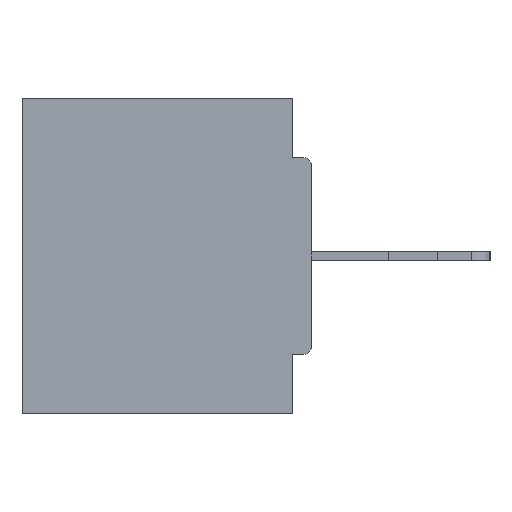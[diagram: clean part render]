
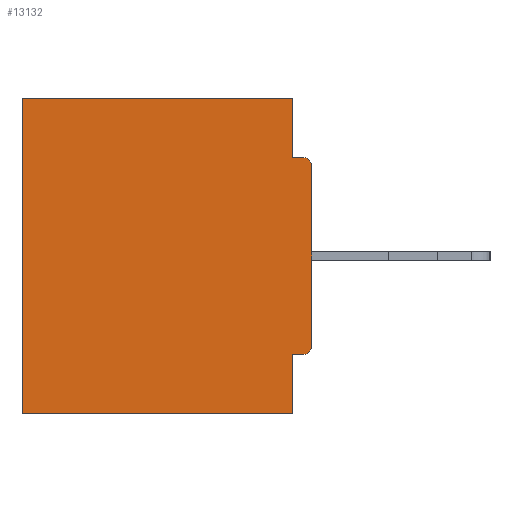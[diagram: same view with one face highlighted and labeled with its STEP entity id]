
A CAD part, left-side view. The second image highlights one B-rep face of the part: STEP entity #13132.
In plain terms, the highlighted planar face has unit normal (-1, 0, 0).
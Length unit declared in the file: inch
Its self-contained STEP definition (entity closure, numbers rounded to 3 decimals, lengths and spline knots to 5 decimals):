
#302 = DIRECTION ( 'NONE',  ( 0., 0., -1. ) ) ;
#1780 = VERTEX_POINT ( 'NONE', #10570 ) ;
#2366 = VERTEX_POINT ( 'NONE', #28621 ) ;
#2694 = LINE ( 'NONE', #25686, #20360 ) ;
#2713 = DIRECTION ( 'NONE',  ( 0., 0., -1. ) ) ;
#3086 = ORIENTED_EDGE ( 'NONE', *, *, #17525, .T. ) ;
#3240 = CARTESIAN_POINT ( 'NONE',  ( 0.298, 0.015, -0.1085 ) ) ;
#3251 = ORIENTED_EDGE ( 'NONE', *, *, #28039, .F. ) ;
#4058 = ORIENTED_EDGE ( 'NONE', *, *, #23724, .F. ) ;
#5071 = CARTESIAN_POINT ( 'NONE',  ( 0.298, 0.031, -0.5 ) ) ;
#5404 = EDGE_CURVE ( 'NONE', #2366, #26169, #7298, .T. ) ;
#5923 = AXIS2_PLACEMENT_3D ( 'NONE', #3240, #13696, #24022 ) ;
#6065 = CARTESIAN_POINT ( 'NONE',  ( 0.298, 0.46, 0. ) ) ;
#6182 = VECTOR ( 'NONE', #30196, 39.37008 ) ;
#6860 = LINE ( 'NONE', #17174, #6182 ) ;
#6928 = CARTESIAN_POINT ( 'NONE',  ( 0.298, 0., -0.3915 ) ) ;
#7298 = LINE ( 'NONE', #27934, #16005 ) ;
#7445 = VERTEX_POINT ( 'NONE', #14035 ) ;
#7808 = VERTEX_POINT ( 'NONE', #9092 ) ;
#9092 = CARTESIAN_POINT ( 'NONE',  ( 0.298, 0.015, -0.4065 ) ) ;
#9270 = CIRCLE ( 'NONE', #23283, 0.015 ) ;
#10570 = CARTESIAN_POINT ( 'NONE',  ( 0.298, 0.031, -0.0935 ) ) ;
#10773 = DIRECTION ( 'NONE',  ( 0., 1., 0. ) ) ;
#11004 = ORIENTED_EDGE ( 'NONE', *, *, #5404, .F. ) ;
#11355 = ORIENTED_EDGE ( 'NONE', *, *, #17517, .T. ) ;
#12876 = DIRECTION ( 'NONE',  ( 0., 0., -1. ) ) ;
#13080 = CARTESIAN_POINT ( 'NONE',  ( 0.298, 0., -0.0935 ) ) ;
#13132 = ADVANCED_FACE ( 'NONE', ( #18272 ), #18106, .F. ) ;
#13502 = VERTEX_POINT ( 'NONE', #6928 ) ;
#13691 = EDGE_CURVE ( 'NONE', #7445, #24953, #26862, .T. ) ;
#13696 = DIRECTION ( 'NONE',  ( -1., 0., 0. ) ) ;
#13926 = CARTESIAN_POINT ( 'NONE',  ( 0.298, 0., -0.1085 ) ) ;
#14035 = CARTESIAN_POINT ( 'NONE',  ( 0.298, 0.46, 0. ) ) ;
#15209 = VECTOR ( 'NONE', #10773, 39.37008 ) ;
#15404 = DIRECTION ( 'NONE',  ( 0., 0., -1. ) ) ;
#15428 = EDGE_CURVE ( 'NONE', #28120, #15691, #16158, .T. ) ;
#15621 = LINE ( 'NONE', #13080, #29986 ) ;
#15691 = VERTEX_POINT ( 'NONE', #18071 ) ;
#15730 = DIRECTION ( 'NONE',  ( 1., 0., 0. ) ) ;
#16005 = VECTOR ( 'NONE', #15404, 39.37008 ) ;
#16012 = EDGE_CURVE ( 'NONE', #28120, #13502, #27368, .T. ) ;
#16090 = ORIENTED_EDGE ( 'NONE', *, *, #15428, .T. ) ;
#16158 = CIRCLE ( 'NONE', #5923, 0.015 ) ;
#16328 = DIRECTION ( 'NONE',  ( -1., 0., 0. ) ) ;
#17174 = CARTESIAN_POINT ( 'NONE',  ( 0.298, 0., -0.4065 ) ) ;
#17517 = EDGE_CURVE ( 'NONE', #28560, #7445, #23941, .T. ) ;
#17525 = EDGE_CURVE ( 'NONE', #7808, #13502, #9270, .T. ) ;
#18071 = CARTESIAN_POINT ( 'NONE',  ( 0.298, 0.015, -0.0935 ) ) ;
#18106 = PLANE ( 'NONE',  #21840 ) ;
#18272 = FACE_OUTER_BOUND ( 'NONE', #26067, .T. ) ;
#18381 = CARTESIAN_POINT ( 'NONE',  ( 0.298, 0.015, -0.3915 ) ) ;
#19358 = CARTESIAN_POINT ( 'NONE',  ( 0.298, 0.031, -0.5 ) ) ;
#20360 = VECTOR ( 'NONE', #26173, 39.37008 ) ;
#20470 = LINE ( 'NONE', #5071, #22951 ) ;
#20626 = CARTESIAN_POINT ( 'NONE',  ( 0.298, 0.46, -0.5 ) ) ;
#20823 = CARTESIAN_POINT ( 'NONE',  ( 0.298, 0.031, 0. ) ) ;
#21840 = AXIS2_PLACEMENT_3D ( 'NONE', #31146, #15730, #12876 ) ;
#22876 = DIRECTION ( 'NONE',  ( 0., -1., 0. ) ) ;
#22950 = ORIENTED_EDGE ( 'NONE', *, *, #30964, .F. ) ;
#22951 = VECTOR ( 'NONE', #2713, 39.37008 ) ;
#23283 = AXIS2_PLACEMENT_3D ( 'NONE', #18381, #16328, #302 ) ;
#23724 = EDGE_CURVE ( 'NONE', #28560, #1780, #20470, .T. ) ;
#23941 = LINE ( 'NONE', #26493, #15209 ) ;
#24022 = DIRECTION ( 'NONE',  ( 0., 0., -1. ) ) ;
#24953 = VERTEX_POINT ( 'NONE', #20626 ) ;
#25686 = CARTESIAN_POINT ( 'NONE',  ( 0.298, 0., -0.5 ) ) ;
#26067 = EDGE_LOOP ( 'NONE', ( #16090, #3251, #4058, #11355, #30776, #22950, #11004, #28220, #3086, #27987 ) ) ;
#26169 = VERTEX_POINT ( 'NONE', #19358 ) ;
#26173 = DIRECTION ( 'NONE',  ( 0., 1., 0. ) ) ;
#26493 = CARTESIAN_POINT ( 'NONE',  ( 0.298, 0., 0. ) ) ;
#26862 = LINE ( 'NONE', #6065, #32166 ) ;
#27368 = LINE ( 'NONE', #29883, #29705 ) ;
#27934 = CARTESIAN_POINT ( 'NONE',  ( 0.298, 0.031, -0.5 ) ) ;
#27987 = ORIENTED_EDGE ( 'NONE', *, *, #16012, .F. ) ;
#28039 = EDGE_CURVE ( 'NONE', #1780, #15691, #15621, .T. ) ;
#28120 = VERTEX_POINT ( 'NONE', #13926 ) ;
#28220 = ORIENTED_EDGE ( 'NONE', *, *, #29136, .F. ) ;
#28560 = VERTEX_POINT ( 'NONE', #20823 ) ;
#28621 = CARTESIAN_POINT ( 'NONE',  ( 0.298, 0.031, -0.4065 ) ) ;
#29136 = EDGE_CURVE ( 'NONE', #7808, #2366, #6860, .T. ) ;
#29389 = DIRECTION ( 'NONE',  ( 0., 0., -1. ) ) ;
#29705 = VECTOR ( 'NONE', #29389, 39.37008 ) ;
#29883 = CARTESIAN_POINT ( 'NONE',  ( 0.298, 0., 0. ) ) ;
#29986 = VECTOR ( 'NONE', #22876, 39.37008 ) ;
#30196 = DIRECTION ( 'NONE',  ( 0., 1., 0. ) ) ;
#30776 = ORIENTED_EDGE ( 'NONE', *, *, #13691, .T. ) ;
#30964 = EDGE_CURVE ( 'NONE', #26169, #24953, #2694, .T. ) ;
#31146 = CARTESIAN_POINT ( 'NONE',  ( 0.298, 0., 0. ) ) ;
#32099 = DIRECTION ( 'NONE',  ( 0., 0., -1. ) ) ;
#32166 = VECTOR ( 'NONE', #32099, 39.37008 ) ;
